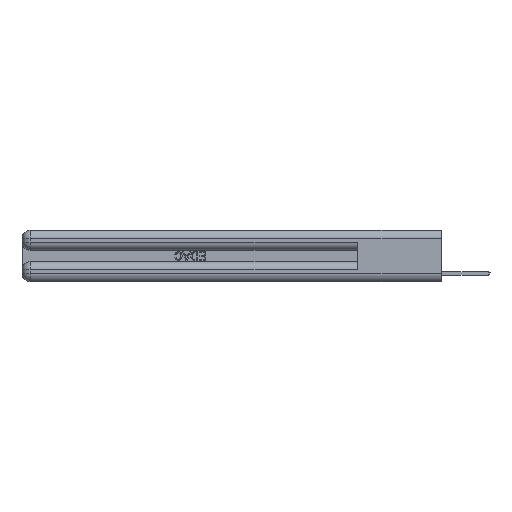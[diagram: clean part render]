
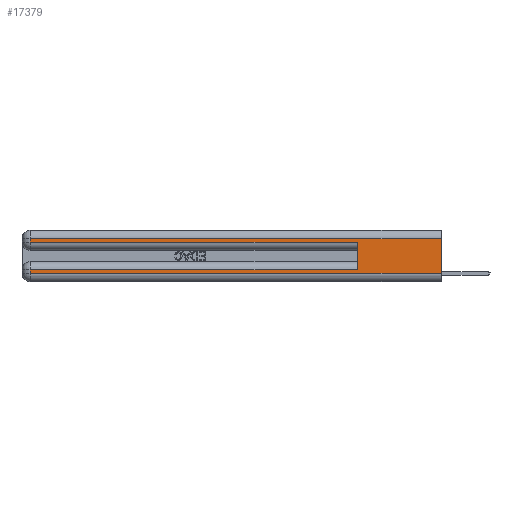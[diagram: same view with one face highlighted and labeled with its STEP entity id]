
A CAD part, left-side view. The second image highlights one B-rep face of the part: STEP entity #17379.
In plain terms, the highlighted planar face has unit normal (-1, 0, 0).
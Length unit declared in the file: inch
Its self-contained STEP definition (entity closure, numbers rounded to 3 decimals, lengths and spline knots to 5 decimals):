
#189 = AXIS2_PLACEMENT_3D ( 'NONE', #636, #21630, #4498 ) ;
#636 = CARTESIAN_POINT ( 'NONE',  ( 0., 0., 0.37 ) ) ;
#1020 = LINE ( 'NONE', #11756, #6701 ) ;
#1273 = VECTOR ( 'NONE', #23590, 39.37008 ) ;
#1340 = EDGE_CURVE ( 'NONE', #11437, #22646, #3083, .T. ) ;
#2618 = CARTESIAN_POINT ( 'NONE',  ( 0., 0., 0.06 ) ) ;
#3083 = LINE ( 'NONE', #22822, #20558 ) ;
#3188 = VERTEX_POINT ( 'NONE', #10370 ) ;
#3322 = CARTESIAN_POINT ( 'NONE',  ( 0., 0., 0.285 ) ) ;
#3347 = ORIENTED_EDGE ( 'NONE', *, *, #25928, .F. ) ;
#3642 = CARTESIAN_POINT ( 'NONE',  ( 0., 0.6, 0.285 ) ) ;
#3887 = EDGE_CURVE ( 'NONE', #9113, #3188, #7136, .T. ) ;
#3977 = VECTOR ( 'NONE', #18919, 39.37008 ) ;
#4498 = DIRECTION ( 'NONE',  ( 0., 0., -1. ) ) ;
#6343 = ORIENTED_EDGE ( 'NONE', *, *, #17818, .T. ) ;
#6355 = CARTESIAN_POINT ( 'NONE',  ( 0., 0.6, 0.085 ) ) ;
#6701 = VECTOR ( 'NONE', #11628, 39.37008 ) ;
#7136 = LINE ( 'NONE', #7529, #19826 ) ;
#7529 = CARTESIAN_POINT ( 'NONE',  ( 0., 0., 0.085 ) ) ;
#8050 = ORIENTED_EDGE ( 'NONE', *, *, #21755, .T. ) ;
#8576 = VECTOR ( 'NONE', #9005, 39.37008 ) ;
#9005 = DIRECTION ( 'NONE',  ( 0., -1., 0. ) ) ;
#9113 = VERTEX_POINT ( 'NONE', #6355 ) ;
#9603 = VECTOR ( 'NONE', #17139, 39.37008 ) ;
#10370 = CARTESIAN_POINT ( 'NONE',  ( 0., 2.94, 0.085 ) ) ;
#10375 = ORIENTED_EDGE ( 'NONE', *, *, #22714, .T. ) ;
#11437 = VERTEX_POINT ( 'NONE', #19128 ) ;
#11628 = DIRECTION ( 'NONE',  ( 0., 0., 1. ) ) ;
#11701 = EDGE_CURVE ( 'NONE', #25090, #14217, #18653, .T. ) ;
#11756 = CARTESIAN_POINT ( 'NONE',  ( 0., 0.6, 0.145 ) ) ;
#12629 = FACE_OUTER_BOUND ( 'NONE', #13008, .T. ) ;
#12846 = LINE ( 'NONE', #2618, #9603 ) ;
#12991 = ORIENTED_EDGE ( 'NONE', *, *, #21666, .T. ) ;
#13008 = EDGE_LOOP ( 'NONE', ( #24259, #10375, #25664, #6343, #3347, #19756, #12991, #8050 ) ) ;
#14217 = VERTEX_POINT ( 'NONE', #23021 ) ;
#14658 = CARTESIAN_POINT ( 'NONE',  ( 0., 2.94, 0.37 ) ) ;
#15536 = CARTESIAN_POINT ( 'NONE',  ( 0., 0., 0.37 ) ) ;
#16582 = DIRECTION ( 'NONE',  ( 0., 0., -1. ) ) ;
#17139 = DIRECTION ( 'NONE',  ( 0., -1., 0. ) ) ;
#17379 = ADVANCED_FACE ( 'NONE', ( #12629 ), #21498, .F. ) ;
#17818 = EDGE_CURVE ( 'NONE', #22646, #22892, #25892, .T. ) ;
#18387 = LINE ( 'NONE', #14658, #24637 ) ;
#18653 = LINE ( 'NONE', #15536, #3977 ) ;
#18919 = DIRECTION ( 'NONE',  ( 0., 0., -1. ) ) ;
#19128 = CARTESIAN_POINT ( 'NONE',  ( 0., 2.94, 0.31 ) ) ;
#19521 = CARTESIAN_POINT ( 'NONE',  ( 0., 2.94, 0.06 ) ) ;
#19707 = DIRECTION ( 'NONE',  ( 0., 1., 0. ) ) ;
#19756 = ORIENTED_EDGE ( 'NONE', *, *, #3887, .T. ) ;
#19826 = VECTOR ( 'NONE', #19707, 39.37008 ) ;
#20043 = CARTESIAN_POINT ( 'NONE',  ( 0., 0., 0.31 ) ) ;
#20558 = VECTOR ( 'NONE', #25172, 39.37008 ) ;
#21498 = PLANE ( 'NONE',  #189 ) ;
#21630 = DIRECTION ( 'NONE',  ( 1., 0., 0. ) ) ;
#21666 = EDGE_CURVE ( 'NONE', #3188, #23193, #18387, .T. ) ;
#21755 = EDGE_CURVE ( 'NONE', #23193, #14217, #12846, .T. ) ;
#22646 = VERTEX_POINT ( 'NONE', #25797 ) ;
#22714 = EDGE_CURVE ( 'NONE', #25090, #11437, #23186, .T. ) ;
#22822 = CARTESIAN_POINT ( 'NONE',  ( 0., 2.94, 0.37 ) ) ;
#22892 = VERTEX_POINT ( 'NONE', #3642 ) ;
#23021 = CARTESIAN_POINT ( 'NONE',  ( 0., 0., 0.06 ) ) ;
#23186 = LINE ( 'NONE', #23456, #1273 ) ;
#23193 = VERTEX_POINT ( 'NONE', #19521 ) ;
#23456 = CARTESIAN_POINT ( 'NONE',  ( 0., 0., 0.31 ) ) ;
#23590 = DIRECTION ( 'NONE',  ( 0., 1., 0. ) ) ;
#24259 = ORIENTED_EDGE ( 'NONE', *, *, #11701, .F. ) ;
#24637 = VECTOR ( 'NONE', #16582, 39.37008 ) ;
#25090 = VERTEX_POINT ( 'NONE', #20043 ) ;
#25172 = DIRECTION ( 'NONE',  ( 0., 0., -1. ) ) ;
#25664 = ORIENTED_EDGE ( 'NONE', *, *, #1340, .T. ) ;
#25797 = CARTESIAN_POINT ( 'NONE',  ( 0., 2.94, 0.285 ) ) ;
#25892 = LINE ( 'NONE', #3322, #8576 ) ;
#25928 = EDGE_CURVE ( 'NONE', #9113, #22892, #1020, .T. ) ;
